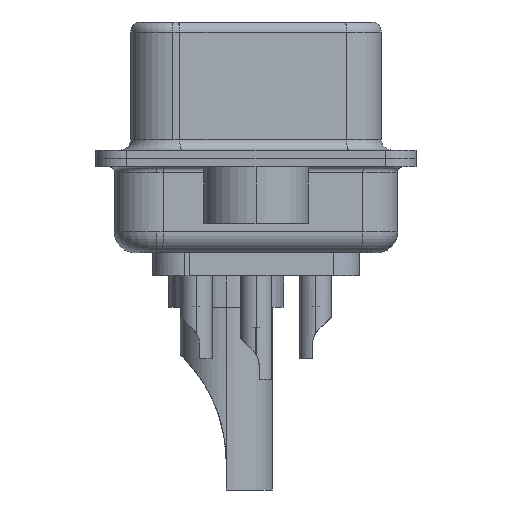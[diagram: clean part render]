
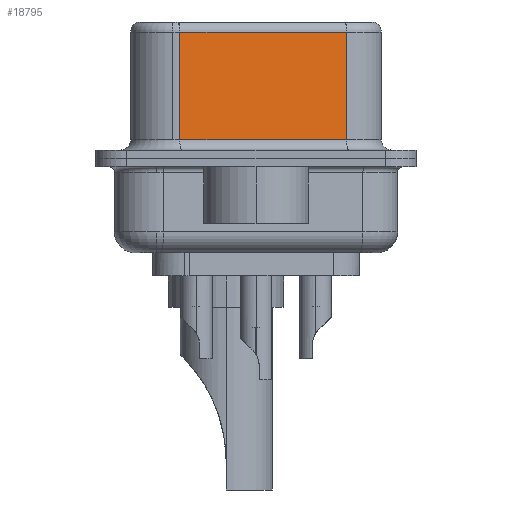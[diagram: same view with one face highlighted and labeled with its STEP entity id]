
A CAD part, left-side view. The second image highlights one B-rep face of the part: STEP entity #18795.
In plain terms, the highlighted planar face has unit normal (-0.985, -0.174, 0).
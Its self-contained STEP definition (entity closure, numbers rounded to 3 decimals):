
#3011 = VECTOR ( 'NONE', #13504, 1000. ) ;
#3688 = LINE ( 'NONE', #24576, #3011 ) ;
#4432 = LINE ( 'NONE', #21292, #21468 ) ;
#4480 = VECTOR ( 'NONE', #13140, 1000. ) ;
#4767 = VERTEX_POINT ( 'NONE', #22666 ) ;
#5567 = CARTESIAN_POINT ( 'NONE',  ( 5.132, -4.322, 6.02 ) ) ;
#5665 = VERTEX_POINT ( 'NONE', #26052 ) ;
#5839 = ORIENTED_EDGE ( 'NONE', *, *, #18712, .T. ) ;
#6487 = ORIENTED_EDGE ( 'NONE', *, *, #15054, .T. ) ;
#10578 = EDGE_CURVE ( 'NONE', #21683, #5665, #22214, .T. ) ;
#11775 = ORIENTED_EDGE ( 'NONE', *, *, #21682, .F. ) ;
#11846 = DIRECTION ( 'NONE',  ( 0.985, 0.174, 0. ) ) ;
#12897 = ORIENTED_EDGE ( 'NONE', *, *, #10578, .T. ) ;
#13099 = EDGE_LOOP ( 'NONE', ( #11775, #12897, #6487, #5839 ) ) ;
#13140 = DIRECTION ( 'NONE',  ( -0.174, 0.985, 0. ) ) ;
#13504 = DIRECTION ( 'NONE',  ( 0., 0., -1. ) ) ;
#13675 = CARTESIAN_POINT ( 'NONE',  ( 5.132, -4.322, 0.9 ) ) ;
#13785 = VERTEX_POINT ( 'NONE', #26754 ) ;
#13935 = VECTOR ( 'NONE', #22533, 1000. ) ;
#14618 = LINE ( 'NONE', #13675, #13935 ) ;
#15054 = EDGE_CURVE ( 'NONE', #5665, #13785, #3688, .T. ) ;
#17409 = AXIS2_PLACEMENT_3D ( 'NONE', #25136, #11846, #27337 ) ;
#17775 = FACE_OUTER_BOUND ( 'NONE', #13099, .T. ) ;
#18712 = EDGE_CURVE ( 'NONE', #13785, #4767, #14618, .T. ) ;
#18795 = ADVANCED_FACE ( 'NONE', ( #17775 ), #27244, .F. ) ;
#18966 = DIRECTION ( 'NONE',  ( 0., 0., -1. ) ) ;
#21292 = CARTESIAN_POINT ( 'NONE',  ( 5.132, -4.322, 6.52 ) ) ;
#21468 = VECTOR ( 'NONE', #18966, 1000. ) ;
#21682 = EDGE_CURVE ( 'NONE', #21683, #4767, #4432, .T. ) ;
#21683 = VERTEX_POINT ( 'NONE', #5567 ) ;
#22214 = LINE ( 'NONE', #28617, #4480 ) ;
#22533 = DIRECTION ( 'NONE',  ( 0.174, -0.985, 0. ) ) ;
#22666 = CARTESIAN_POINT ( 'NONE',  ( 5.132, -4.322, 0.9 ) ) ;
#24576 = CARTESIAN_POINT ( 'NONE',  ( 3.73, 3.628, 6.52 ) ) ;
#25136 = CARTESIAN_POINT ( 'NONE',  ( 5.132, -4.322, 6.52 ) ) ;
#26052 = CARTESIAN_POINT ( 'NONE',  ( 3.73, 3.628, 6.02 ) ) ;
#26754 = CARTESIAN_POINT ( 'NONE',  ( 3.73, 3.628, 0.9 ) ) ;
#27244 = PLANE ( 'NONE',  #17409 ) ;
#27337 = DIRECTION ( 'NONE',  ( -0.174, 0.985, 0. ) ) ;
#28617 = CARTESIAN_POINT ( 'NONE',  ( 5.132, -4.322, 6.02 ) ) ;
